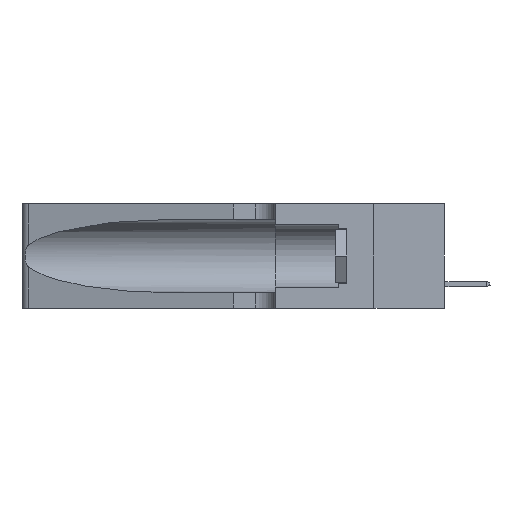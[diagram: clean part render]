
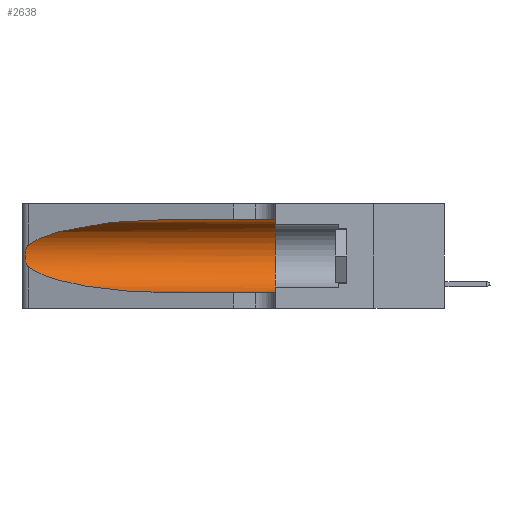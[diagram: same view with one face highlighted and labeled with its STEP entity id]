
A CAD part, left-side view. The second image highlights one B-rep face of the part: STEP entity #2638.
In plain terms, the highlighted cylindrical face has radius 3.308 mm (diameter 6.617 mm), a partial arc.
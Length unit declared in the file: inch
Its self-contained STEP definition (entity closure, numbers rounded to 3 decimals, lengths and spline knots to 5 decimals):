
#131 = ORIENTED_EDGE ( 'NONE', *, *, #19484, .F. ) ;
#148 = DIRECTION ( 'NONE',  ( 0., -1., 0. ) ) ;
#308 = CARTESIAN_POINT ( 'NONE',  ( 0.1305, 1.61858, 0.31525 ) ) ;
#392 = B_SPLINE_CURVE_WITH_KNOTS ( 'NONE', 3,
 ( #16311, #4417, #23888, #12135, #2821, #16393, #2469, #16067, #18001, #6381, #580, #14797, #929, #5179 ),
 .UNSPECIFIED., .F., .F.,
 ( 4, 2, 2, 2, 2, 2, 4 ),
 ( 0., 0.00027, 0.00053, 0.00107, 0.0016, 0.00187, 0.00214 ),
 .UNSPECIFIED. ) ;
#580 = CARTESIAN_POINT ( 'NONE',  ( 0.25789, 1.23486, 0.15765 ) ) ;
#929 = CARTESIAN_POINT ( 'NONE',  ( 0.25555, 1.22993, 0.14849 ) ) ;
#1081 = ORIENTED_EDGE ( 'NONE', *, *, #11244, .T. ) ;
#1544 = DIRECTION ( 'NONE',  ( 0., -1., 0. ) ) ;
#2206 = VECTOR ( 'NONE', #148, 39.37008 ) ;
#2469 = CARTESIAN_POINT ( 'NONE',  ( 0.26075, 1.23896, 0.19203 ) ) ;
#2523 = LINE ( 'NONE', #5372, #17388 ) ;
#2572 = CARTESIAN_POINT ( 'NONE',  ( 0.2373, 1.15595, 0.08982 ) ) ;
#2638 = ADVANCED_FACE ( 'NONE', ( #17312 ), #5176, .F. ) ;
#2821 = CARTESIAN_POINT ( 'NONE',  ( 0.25854, 1.2359, 0.20912 ) ) ;
#4299 =( BOUNDED_CURVE ( )  B_SPLINE_CURVE ( 3, ( #11009, #22758, #24686, #16926 ),
 .UNSPECIFIED., .F., .F. ) 
 B_SPLINE_CURVE_WITH_KNOTS ( ( 4, 4 ),
 ( 1.5708, 2.84003 ),
 .UNSPECIFIED. ) 
 CURVE ( )  GEOMETRIC_REPRESENTATION_ITEM ( )  RATIONAL_B_SPLINE_CURVE ( ( 1., 0.87, 0.87, 1. ) ) 
 REPRESENTATION_ITEM ( '' )  );
#4417 = CARTESIAN_POINT ( 'NONE',  ( 0.25555, 1.22994, 0.2215 ) ) ;
#4698 = CARTESIAN_POINT ( 'NONE',  ( 0.18966, 0.96281, 0.05475 ) ) ;
#5176 = CYLINDRICAL_SURFACE ( 'NONE', #23607, 0.13025 ) ;
#5179 = CARTESIAN_POINT ( 'NONE',  ( 0.25487, 1.22718, 0.14631 ) ) ;
#5372 = CARTESIAN_POINT ( 'NONE',  ( 0.1305, 1.61858, 0.05475 ) ) ;
#5861 = LINE ( 'NONE', #308, #2206 ) ;
#5947 = EDGE_CURVE ( 'NONE', #11547, #24568, #8684, .T. ) ;
#6381 = CARTESIAN_POINT ( 'NONE',  ( 0.25856, 1.23593, 0.16098 ) ) ;
#6832 = DIRECTION ( 'NONE',  ( 0., 0., -1. ) ) ;
#6916 = EDGE_LOOP ( 'NONE', ( #22944, #25017, #1081, #12031, #12926, #131 ) ) ;
#8112 = VERTEX_POINT ( 'NONE', #17764 ) ;
#8684 = CIRCLE ( 'NONE', #13067, 0.13025 ) ;
#8698 = CARTESIAN_POINT ( 'NONE',  ( 0.25487, 1.22718, 0.14631 ) ) ;
#11009 = CARTESIAN_POINT ( 'NONE',  ( 0.1305, 0.72297, 0.31525 ) ) ;
#11244 = EDGE_CURVE ( 'NONE', #23276, #23532, #22725, .T. ) ;
#11547 = VERTEX_POINT ( 'NONE', #19804 ) ;
#11953 = CARTESIAN_POINT ( 'NONE',  ( 0.1305, 0.35, 0.05475 ) ) ;
#12031 = ORIENTED_EDGE ( 'NONE', *, *, #19529, .T. ) ;
#12135 = CARTESIAN_POINT ( 'NONE',  ( 0.25787, 1.23484, 0.2124 ) ) ;
#12926 = ORIENTED_EDGE ( 'NONE', *, *, #5947, .F. ) ;
#13067 = AXIS2_PLACEMENT_3D ( 'NONE', #20302, #22272, #14947 ) ;
#14797 = CARTESIAN_POINT ( 'NONE',  ( 0.25639, 1.23186, 0.15144 ) ) ;
#14947 = DIRECTION ( 'NONE',  ( 0., 0., 1. ) ) ;
#16067 = CARTESIAN_POINT ( 'NONE',  ( 0.26075, 1.23896, 0.178 ) ) ;
#16311 = CARTESIAN_POINT ( 'NONE',  ( 0.25487, 1.22718, 0.22369 ) ) ;
#16393 = CARTESIAN_POINT ( 'NONE',  ( 0.26018, 1.23835, 0.19895 ) ) ;
#16926 = CARTESIAN_POINT ( 'NONE',  ( 0.25487, 1.22718, 0.22369 ) ) ;
#17198 = EDGE_CURVE ( 'NONE', #19029, #23276, #392, .T. ) ;
#17233 = DIRECTION ( 'NONE',  ( 0., -1., 0. ) ) ;
#17312 = FACE_OUTER_BOUND ( 'NONE', #6916, .T. ) ;
#17388 = VECTOR ( 'NONE', #17233, 39.37008 ) ;
#17478 = CARTESIAN_POINT ( 'NONE',  ( 0.25487, 1.22718, 0.14631 ) ) ;
#17764 = CARTESIAN_POINT ( 'NONE',  ( 0.1305, 0.72297, 0.31525 ) ) ;
#18001 = CARTESIAN_POINT ( 'NONE',  ( 0.26017, 1.23833, 0.17102 ) ) ;
#19029 = VERTEX_POINT ( 'NONE', #24485 ) ;
#19484 = EDGE_CURVE ( 'NONE', #8112, #11547, #5861, .T. ) ;
#19529 = EDGE_CURVE ( 'NONE', #23532, #24568, #2523, .T. ) ;
#19804 = CARTESIAN_POINT ( 'NONE',  ( 0.1305, 0.35, 0.31525 ) ) ;
#20302 = CARTESIAN_POINT ( 'NONE',  ( 0.1305, 0.35, 0.185 ) ) ;
#20829 = EDGE_CURVE ( 'NONE', #8112, #19029, #4299, .T. ) ;
#21772 = CARTESIAN_POINT ( 'NONE',  ( 0.1305, 0.72297, 0.05475 ) ) ;
#22272 = DIRECTION ( 'NONE',  ( 0., 1., 0. ) ) ;
#22725 =( BOUNDED_CURVE ( )  B_SPLINE_CURVE ( 3, ( #8698, #2572, #4698, #23993 ),
 .UNSPECIFIED., .F., .F. ) 
 B_SPLINE_CURVE_WITH_KNOTS ( ( 4, 4 ),
 ( 3.44316, 4.71239 ),
 .UNSPECIFIED. ) 
 CURVE ( )  GEOMETRIC_REPRESENTATION_ITEM ( )  RATIONAL_B_SPLINE_CURVE ( ( 1., 0.87, 0.87, 1. ) ) 
 REPRESENTATION_ITEM ( '' )  );
#22758 = CARTESIAN_POINT ( 'NONE',  ( 0.18966, 0.96281, 0.31525 ) ) ;
#22944 = ORIENTED_EDGE ( 'NONE', *, *, #20829, .T. ) ;
#23276 = VERTEX_POINT ( 'NONE', #17478 ) ;
#23532 = VERTEX_POINT ( 'NONE', #21772 ) ;
#23607 = AXIS2_PLACEMENT_3D ( 'NONE', #24178, #1544, #6832 ) ;
#23888 = CARTESIAN_POINT ( 'NONE',  ( 0.25639, 1.23184, 0.21858 ) ) ;
#23993 = CARTESIAN_POINT ( 'NONE',  ( 0.1305, 0.72297, 0.05475 ) ) ;
#24178 = CARTESIAN_POINT ( 'NONE',  ( 0.1305, 1.61858, 0.185 ) ) ;
#24485 = CARTESIAN_POINT ( 'NONE',  ( 0.25487, 1.22718, 0.22369 ) ) ;
#24568 = VERTEX_POINT ( 'NONE', #11953 ) ;
#24686 = CARTESIAN_POINT ( 'NONE',  ( 0.2373, 1.15595, 0.28018 ) ) ;
#25017 = ORIENTED_EDGE ( 'NONE', *, *, #17198, .T. ) ;
